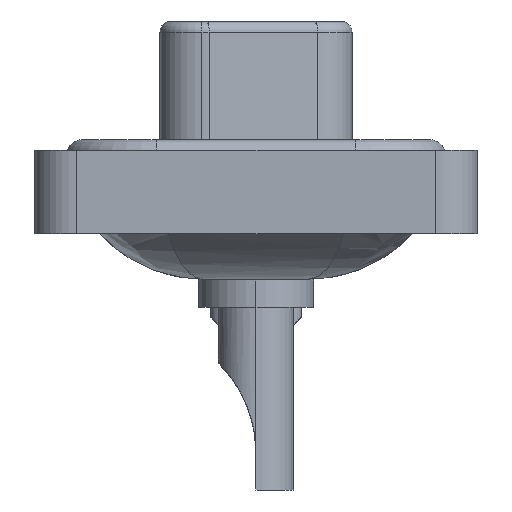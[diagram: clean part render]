
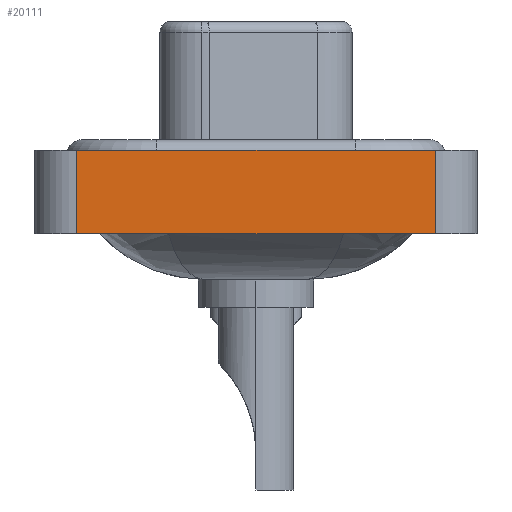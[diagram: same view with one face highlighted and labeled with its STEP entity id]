
A CAD part, left-side view. The second image highlights one B-rep face of the part: STEP entity #20111.
In plain terms, the highlighted planar face has unit normal (-1, 0, 0).
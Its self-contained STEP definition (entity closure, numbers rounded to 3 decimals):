
#867 = LINE ( 'NONE', #15617, #15497 ) ;
#1060 = EDGE_LOOP ( 'NONE', ( #18511, #3877, #14591, #17700 ) ) ;
#1706 = LINE ( 'NONE', #8907, #19232 ) ;
#1893 = CARTESIAN_POINT ( 'NONE',  ( -7.35, -8.55, -3.6 ) ) ;
#2191 = VECTOR ( 'NONE', #5428, 1000. ) ;
#3646 = CARTESIAN_POINT ( 'NONE',  ( -7.35, 8.55, -3.6 ) ) ;
#3877 = ORIENTED_EDGE ( 'NONE', *, *, #11038, .F. ) ;
#4067 = DIRECTION ( 'NONE',  ( -1., 0., 0. ) ) ;
#4273 = VERTEX_POINT ( 'NONE', #19185 ) ;
#4300 = FACE_OUTER_BOUND ( 'NONE', #1060, .T. ) ;
#5070 = VERTEX_POINT ( 'NONE', #1893 ) ;
#5428 = DIRECTION ( 'NONE',  ( 0., -1., 0. ) ) ;
#7683 = LINE ( 'NONE', #14531, #2191 ) ;
#7848 = PLANE ( 'NONE',  #16662 ) ;
#8802 = EDGE_CURVE ( 'NONE', #19767, #4273, #1706, .T. ) ;
#8907 = CARTESIAN_POINT ( 'NONE',  ( -7.35, 8.55, -3.6 ) ) ;
#9860 = DIRECTION ( 'NONE',  ( 0., 0., 1. ) ) ;
#11038 = EDGE_CURVE ( 'NONE', #4273, #14789, #7683, .T. ) ;
#11975 = DIRECTION ( 'NONE',  ( 0., -1., 0. ) ) ;
#12243 = DIRECTION ( 'NONE',  ( 0., 0., 1. ) ) ;
#13394 = CARTESIAN_POINT ( 'NONE',  ( -7.35, -8.55, -3.6 ) ) ;
#13739 = CARTESIAN_POINT ( 'NONE',  ( -7.35, -8.55, -3.6 ) ) ;
#14531 = CARTESIAN_POINT ( 'NONE',  ( -7.35, -8.55, 0.4 ) ) ;
#14591 = ORIENTED_EDGE ( 'NONE', *, *, #8802, .F. ) ;
#14789 = VERTEX_POINT ( 'NONE', #16483 ) ;
#15164 = DIRECTION ( 'NONE',  ( 0., 0., 1. ) ) ;
#15497 = VECTOR ( 'NONE', #11975, 1000. ) ;
#15617 = CARTESIAN_POINT ( 'NONE',  ( -7.35, -8.55, -3.6 ) ) ;
#16483 = CARTESIAN_POINT ( 'NONE',  ( -7.35, -8.55, 0.4 ) ) ;
#16662 = AXIS2_PLACEMENT_3D ( 'NONE', #13394, #4067, #15164 ) ;
#17700 = ORIENTED_EDGE ( 'NONE', *, *, #18957, .T. ) ;
#18511 = ORIENTED_EDGE ( 'NONE', *, *, #18925, .T. ) ;
#18822 = LINE ( 'NONE', #13739, #21543 ) ;
#18925 = EDGE_CURVE ( 'NONE', #5070, #14789, #18822, .T. ) ;
#18957 = EDGE_CURVE ( 'NONE', #19767, #5070, #867, .T. ) ;
#19185 = CARTESIAN_POINT ( 'NONE',  ( -7.35, 8.55, 0.4 ) ) ;
#19232 = VECTOR ( 'NONE', #12243, 1000. ) ;
#19767 = VERTEX_POINT ( 'NONE', #3646 ) ;
#20111 = ADVANCED_FACE ( 'NONE', ( #4300 ), #7848, .T. ) ;
#21543 = VECTOR ( 'NONE', #9860, 1000. ) ;
